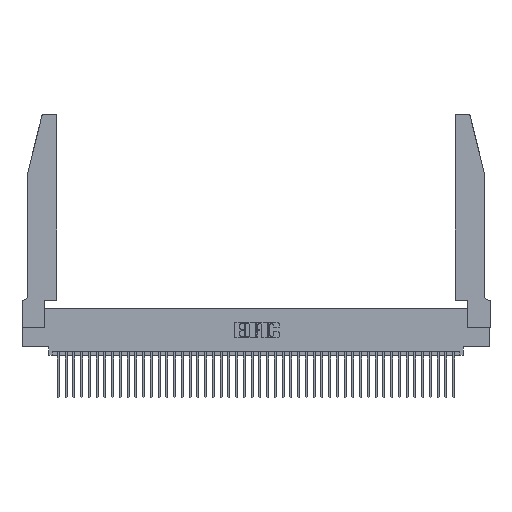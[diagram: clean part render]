
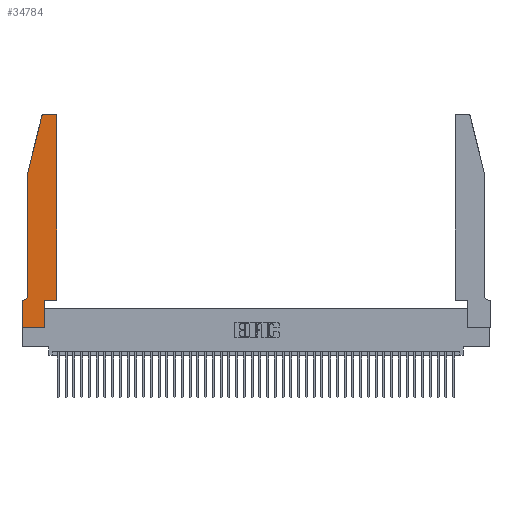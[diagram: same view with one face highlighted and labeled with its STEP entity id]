
A CAD part, top view. The second image highlights one B-rep face of the part: STEP entity #34784.
In plain terms, the highlighted planar face has unit normal (0, 0, 1).
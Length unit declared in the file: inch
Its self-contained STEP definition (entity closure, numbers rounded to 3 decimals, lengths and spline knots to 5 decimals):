
#365 = VERTEX_POINT ( 'NONE', #1095 ) ;
#696 = DIRECTION ( 'NONE',  ( 0., 1., 0. ) ) ;
#745 = DIRECTION ( 'NONE',  ( 0., 0., 1. ) ) ;
#1017 = EDGE_CURVE ( 'NONE', #1686, #24011, #29167, .T. ) ;
#1095 = CARTESIAN_POINT ( 'NONE',  ( 0., 0.35, 0.37 ) ) ;
#1686 = VERTEX_POINT ( 'NONE', #15916 ) ;
#2213 = DIRECTION ( 'NONE',  ( 1., 0., 0. ) ) ;
#2215 = ORIENTED_EDGE ( 'NONE', *, *, #27575, .T. ) ;
#2248 = CARTESIAN_POINT ( 'NONE',  ( 0.4505, 0.35, 0.37 ) ) ;
#2609 = EDGE_CURVE ( 'NONE', #365, #3456, #22655, .T. ) ;
#3456 = VERTEX_POINT ( 'NONE', #41804 ) ;
#4111 = LINE ( 'NONE', #13954, #20355 ) ;
#4270 = VECTOR ( 'NONE', #17345, 39.37008 ) ;
#5928 = DIRECTION ( 'NONE',  ( 1., 0., 0. ) ) ;
#6218 = CARTESIAN_POINT ( 'NONE',  ( 0.2605, 2.75, 0.37 ) ) ;
#6807 = VERTEX_POINT ( 'NONE', #9300 ) ;
#7747 = LINE ( 'NONE', #36666, #40793 ) ;
#7992 = EDGE_CURVE ( 'NONE', #21864, #17557, #34602, .T. ) ;
#8067 = AXIS2_PLACEMENT_3D ( 'NONE', #31483, #11042, #34856 ) ;
#8825 = VECTOR ( 'NONE', #39008, 39.37008 ) ;
#9300 = CARTESIAN_POINT ( 'NONE',  ( 0.284, 2.75, 0.37 ) ) ;
#9767 = DIRECTION ( 'NONE',  ( -1., 0., 0. ) ) ;
#11042 = DIRECTION ( 'NONE',  ( 0., 0., 1. ) ) ;
#11525 = ORIENTED_EDGE ( 'NONE', *, *, #2609, .T. ) ;
#12080 = ORIENTED_EDGE ( 'NONE', *, *, #37524, .T. ) ;
#12184 = CARTESIAN_POINT ( 'NONE',  ( 0.4505, 2.72, 0.37 ) ) ;
#12212 = DIRECTION ( 'NONE',  ( 0., 1., 0. ) ) ;
#12381 = EDGE_CURVE ( 'NONE', #3456, #15456, #16139, .T. ) ;
#12869 = DIRECTION ( 'NONE',  ( -1., 0., 0. ) ) ;
#13121 = ORIENTED_EDGE ( 'NONE', *, *, #1017, .T. ) ;
#13954 = CARTESIAN_POINT ( 'NONE',  ( 0.0755, 2., 0.37 ) ) ;
#14074 = CIRCLE ( 'NONE', #16319, 0.07 ) ;
#14360 = VERTEX_POINT ( 'NONE', #25154 ) ;
#14662 = VECTOR ( 'NONE', #9767, 39.37008 ) ;
#14971 = EDGE_CURVE ( 'NONE', #6807, #1686, #44048, .T. ) ;
#15070 = VECTOR ( 'NONE', #2213, 39.37008 ) ;
#15456 = VERTEX_POINT ( 'NONE', #17595 ) ;
#15916 = CARTESIAN_POINT ( 'NONE',  ( 0.25487, 2.72718, 0.37 ) ) ;
#16139 = LINE ( 'NONE', #43190, #15070 ) ;
#16221 = CARTESIAN_POINT ( 'NONE',  ( 0.0055, 0.42, 0.37 ) ) ;
#16319 = AXIS2_PLACEMENT_3D ( 'NONE', #16221, #40022, #19708 ) ;
#16745 = CARTESIAN_POINT ( 'NONE',  ( 0.0055, 0.35, 0.37 ) ) ;
#17345 = DIRECTION ( 'NONE',  ( 0., -1., 0. ) ) ;
#17557 = VERTEX_POINT ( 'NONE', #12184 ) ;
#17576 = EDGE_LOOP ( 'NONE', ( #27005, #35989, #13121, #43402, #37602, #2215, #11525, #22782, #31791, #40784, #17943, #12080 ) ) ;
#17595 = CARTESIAN_POINT ( 'NONE',  ( 0.2865, 0., 0.37 ) ) ;
#17887 = LINE ( 'NONE', #6218, #14662 ) ;
#17943 = ORIENTED_EDGE ( 'NONE', *, *, #7992, .T. ) ;
#18070 = DIRECTION ( 'NONE',  ( 0., 0., 1. ) ) ;
#18545 = CIRCLE ( 'NONE', #43208, 0.03 ) ;
#19708 = DIRECTION ( 'NONE',  ( -1., 0., 0. ) ) ;
#19802 = LINE ( 'NONE', #22405, #36796 ) ;
#20355 = VECTOR ( 'NONE', #24258, 39.37008 ) ;
#21025 = EDGE_CURVE ( 'NONE', #23916, #36476, #14074, .T. ) ;
#21234 = PLANE ( 'NONE',  #8067 ) ;
#21529 = CARTESIAN_POINT ( 'NONE',  ( 0.284, 2.72, 0.37 ) ) ;
#21864 = VERTEX_POINT ( 'NONE', #24274 ) ;
#22405 = CARTESIAN_POINT ( 'NONE',  ( 0.2865, 0.35, 0.37 ) ) ;
#22655 = LINE ( 'NONE', #34179, #4270 ) ;
#22733 = EDGE_CURVE ( 'NONE', #24011, #23916, #4111, .T. ) ;
#22782 = ORIENTED_EDGE ( 'NONE', *, *, #12381, .T. ) ;
#23916 = VERTEX_POINT ( 'NONE', #31150 ) ;
#24011 = VERTEX_POINT ( 'NONE', #24759 ) ;
#24258 = DIRECTION ( 'NONE',  ( 0., -1., 0. ) ) ;
#24274 = CARTESIAN_POINT ( 'NONE',  ( 0.4505, 0.35, 0.37 ) ) ;
#24338 = EDGE_CURVE ( 'NONE', #14360, #21864, #26650, .T. ) ;
#24501 = VECTOR ( 'NONE', #5928, 39.37008 ) ;
#24759 = CARTESIAN_POINT ( 'NONE',  ( 0.0755, 2., 0.37 ) ) ;
#24804 = AXIS2_PLACEMENT_3D ( 'NONE', #21529, #745, #24947 ) ;
#24947 = DIRECTION ( 'NONE',  ( 1., 0., 0. ) ) ;
#25055 = CARTESIAN_POINT ( 'NONE',  ( 0.4505, 0.35, 0.37 ) ) ;
#25154 = CARTESIAN_POINT ( 'NONE',  ( 0.2865, 0.35, 0.37 ) ) ;
#26650 = LINE ( 'NONE', #2248, #24501 ) ;
#26681 = VECTOR ( 'NONE', #696, 39.37008 ) ;
#27005 = ORIENTED_EDGE ( 'NONE', *, *, #35830, .T. ) ;
#27082 = FACE_OUTER_BOUND ( 'NONE', #17576, .T. ) ;
#27575 = EDGE_CURVE ( 'NONE', #36476, #365, #7747, .T. ) ;
#29167 = LINE ( 'NONE', #38951, #8825 ) ;
#31150 = CARTESIAN_POINT ( 'NONE',  ( 0.0755, 0.42, 0.37 ) ) ;
#31483 = CARTESIAN_POINT ( 'NONE',  ( 0., 0.35, 0.37 ) ) ;
#31791 = ORIENTED_EDGE ( 'NONE', *, *, #41331, .T. ) ;
#34179 = CARTESIAN_POINT ( 'NONE',  ( 0., 0., 0.37 ) ) ;
#34602 = LINE ( 'NONE', #25055, #26681 ) ;
#34784 = ADVANCED_FACE ( 'NONE', ( #27082 ), #21234, .T. ) ;
#34856 = DIRECTION ( 'NONE',  ( 1., 0., 0. ) ) ;
#35660 = VERTEX_POINT ( 'NONE', #42789 ) ;
#35830 = EDGE_CURVE ( 'NONE', #35660, #6807, #17887, .T. ) ;
#35989 = ORIENTED_EDGE ( 'NONE', *, *, #14971, .T. ) ;
#36476 = VERTEX_POINT ( 'NONE', #16745 ) ;
#36666 = CARTESIAN_POINT ( 'NONE',  ( 0.0755, 0.35, 0.37 ) ) ;
#36796 = VECTOR ( 'NONE', #12212, 39.37008 ) ;
#37524 = EDGE_CURVE ( 'NONE', #17557, #35660, #18545, .T. ) ;
#37602 = ORIENTED_EDGE ( 'NONE', *, *, #21025, .T. ) ;
#38394 = CARTESIAN_POINT ( 'NONE',  ( 0.4205, 2.72, 0.37 ) ) ;
#38951 = CARTESIAN_POINT ( 'NONE',  ( 0.0755, 2., 0.37 ) ) ;
#39008 = DIRECTION ( 'NONE',  ( -0.239, -0.971, 0. ) ) ;
#40022 = DIRECTION ( 'NONE',  ( 0., 0., -1. ) ) ;
#40784 = ORIENTED_EDGE ( 'NONE', *, *, #24338, .T. ) ;
#40793 = VECTOR ( 'NONE', #12869, 39.37008 ) ;
#41331 = EDGE_CURVE ( 'NONE', #15456, #14360, #19802, .T. ) ;
#41804 = CARTESIAN_POINT ( 'NONE',  ( 0., 0., 0.37 ) ) ;
#41817 = DIRECTION ( 'NONE',  ( 1., 0., 0. ) ) ;
#42789 = CARTESIAN_POINT ( 'NONE',  ( 0.4205, 2.75, 0.37 ) ) ;
#43190 = CARTESIAN_POINT ( 'NONE',  ( 0., 0., 0.37 ) ) ;
#43208 = AXIS2_PLACEMENT_3D ( 'NONE', #38394, #18070, #41817 ) ;
#43402 = ORIENTED_EDGE ( 'NONE', *, *, #22733, .T. ) ;
#44048 = CIRCLE ( 'NONE', #24804, 0.03 ) ;
